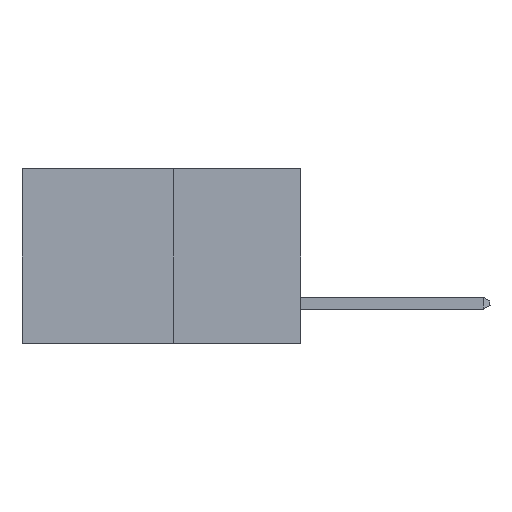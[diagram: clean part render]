
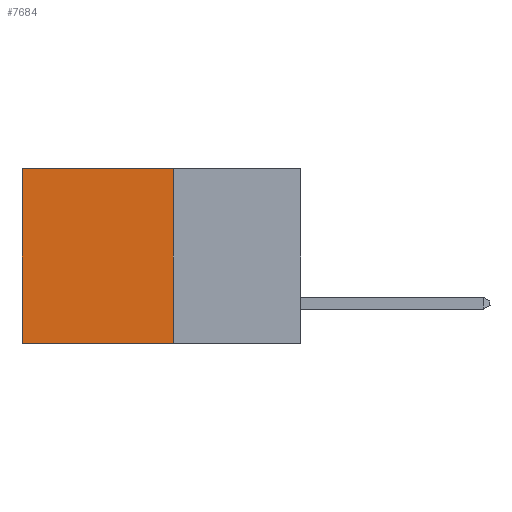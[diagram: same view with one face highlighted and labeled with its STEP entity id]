
A CAD part, left-side view. The second image highlights one B-rep face of the part: STEP entity #7684.
In plain terms, the highlighted planar face has unit normal (-1, 0, 0).
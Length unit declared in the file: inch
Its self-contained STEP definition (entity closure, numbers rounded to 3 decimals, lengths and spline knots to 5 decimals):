
#331 = FACE_OUTER_BOUND ( 'NONE', #16385, .T. ) ;
#959 = VERTEX_POINT ( 'NONE', #19007 ) ;
#1351 = VERTEX_POINT ( 'NONE', #15718 ) ;
#1709 = VERTEX_POINT ( 'NONE', #8139 ) ;
#2805 = VECTOR ( 'NONE', #5403, 39.37008 ) ;
#4064 = EDGE_CURVE ( 'NONE', #9910, #1351, #21809, .T. ) ;
#4999 = CARTESIAN_POINT ( 'NONE',  ( 0.277, 0.27, -0.37 ) ) ;
#5403 = DIRECTION ( 'NONE',  ( 0., 1., 0. ) ) ;
#6083 = PLANE ( 'NONE',  #8325 ) ;
#6514 = ORIENTED_EDGE ( 'NONE', *, *, #4064, .T. ) ;
#6688 = ORIENTED_EDGE ( 'NONE', *, *, #7369, .F. ) ;
#6734 = ORIENTED_EDGE ( 'NONE', *, *, #20216, .F. ) ;
#6976 = ORIENTED_EDGE ( 'NONE', *, *, #11701, .T. ) ;
#7369 = EDGE_CURVE ( 'NONE', #1709, #1351, #12112, .T. ) ;
#7684 = ADVANCED_FACE ( 'NONE', ( #331 ), #6083, .F. ) ;
#7974 = DIRECTION ( 'NONE',  ( 0., 0., -1. ) ) ;
#8139 = CARTESIAN_POINT ( 'NONE',  ( 0.277, 0.27, -0.37 ) ) ;
#8325 = AXIS2_PLACEMENT_3D ( 'NONE', #14820, #18266, #7974 ) ;
#8916 = LINE ( 'NONE', #13358, #17455 ) ;
#9910 = VERTEX_POINT ( 'NONE', #11819 ) ;
#11701 = EDGE_CURVE ( 'NONE', #959, #9910, #18316, .T. ) ;
#11819 = CARTESIAN_POINT ( 'NONE',  ( 0.277, 0.59, 0. ) ) ;
#11874 = CARTESIAN_POINT ( 'NONE',  ( 0.277, 0.27, 0. ) ) ;
#11946 = DIRECTION ( 'NONE',  ( 0., 1., 0. ) ) ;
#12112 = LINE ( 'NONE', #4999, #2805 ) ;
#13358 = CARTESIAN_POINT ( 'NONE',  ( 0.277, 0.27, -0.37 ) ) ;
#14820 = CARTESIAN_POINT ( 'NONE',  ( 0.277, 0.27, -0.37 ) ) ;
#15051 = DIRECTION ( 'NONE',  ( 0., 0., -1. ) ) ;
#15515 = DIRECTION ( 'NONE',  ( 0., 0., -1. ) ) ;
#15718 = CARTESIAN_POINT ( 'NONE',  ( 0.277, 0.59, -0.37 ) ) ;
#16385 = EDGE_LOOP ( 'NONE', ( #6514, #6688, #6734, #6976 ) ) ;
#17455 = VECTOR ( 'NONE', #15051, 39.37008 ) ;
#18266 = DIRECTION ( 'NONE',  ( 1., 0., 0. ) ) ;
#18316 = LINE ( 'NONE', #11874, #22161 ) ;
#18495 = CARTESIAN_POINT ( 'NONE',  ( 0.277, 0.59, -0.37 ) ) ;
#19007 = CARTESIAN_POINT ( 'NONE',  ( 0.277, 0.27, 0. ) ) ;
#20216 = EDGE_CURVE ( 'NONE', #959, #1709, #8916, .T. ) ;
#21312 = VECTOR ( 'NONE', #15515, 39.37008 ) ;
#21809 = LINE ( 'NONE', #18495, #21312 ) ;
#22161 = VECTOR ( 'NONE', #11946, 39.37008 ) ;
